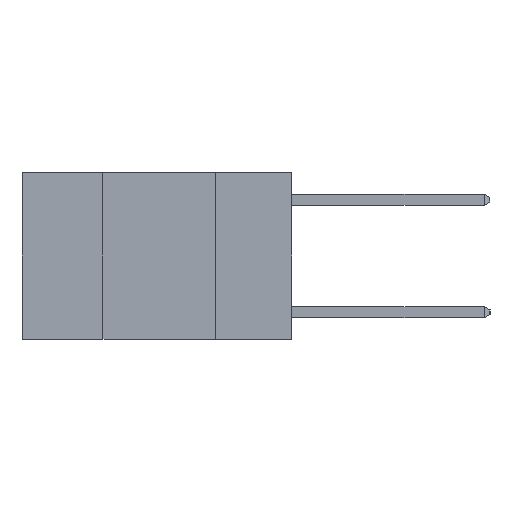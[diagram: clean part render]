
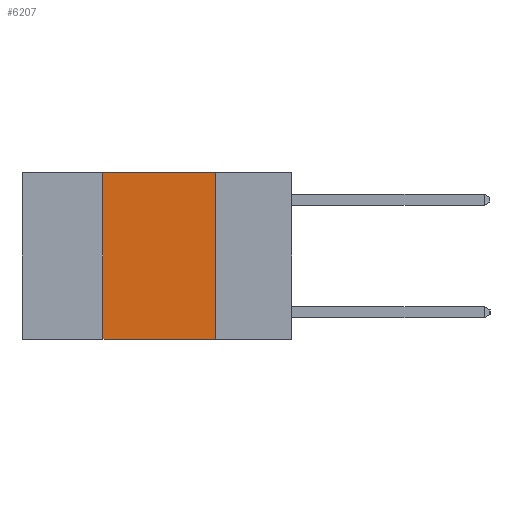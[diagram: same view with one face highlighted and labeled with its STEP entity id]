
A CAD part, left-side view. The second image highlights one B-rep face of the part: STEP entity #6207.
In plain terms, the highlighted planar face has unit normal (-1, 0, 0).
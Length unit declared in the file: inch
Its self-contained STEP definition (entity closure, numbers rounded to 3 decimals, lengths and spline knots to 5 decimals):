
#138 = DIRECTION ( 'NONE',  ( 0., 0., -1. ) ) ;
#323 = EDGE_CURVE ( 'NONE', #2828, #8294, #5029, .T. ) ;
#560 = ORIENTED_EDGE ( 'NONE', *, *, #2396, .F. ) ;
#1161 = LINE ( 'NONE', #9359, #9073 ) ;
#1712 = VERTEX_POINT ( 'NONE', #9080 ) ;
#1921 = VECTOR ( 'NONE', #7247, 39.37008 ) ;
#1958 = DIRECTION ( 'NONE',  ( 0., 0., -1. ) ) ;
#2396 = EDGE_CURVE ( 'NONE', #2738, #1712, #5252, .T. ) ;
#2738 = VERTEX_POINT ( 'NONE', #8018 ) ;
#2828 = VERTEX_POINT ( 'NONE', #9336 ) ;
#2968 = EDGE_CURVE ( 'NONE', #2828, #2738, #4510, .T. ) ;
#3489 = EDGE_CURVE ( 'NONE', #1712, #8294, #1161, .T. ) ;
#3883 = CARTESIAN_POINT ( 'NONE',  ( 0., 0.6, 0. ) ) ;
#4510 = LINE ( 'NONE', #9466, #1921 ) ;
#5029 = LINE ( 'NONE', #9624, #7030 ) ;
#5087 = CARTESIAN_POINT ( 'NONE',  ( 0., 0.6, 0. ) ) ;
#5252 = LINE ( 'NONE', #3883, #8754 ) ;
#6102 = CARTESIAN_POINT ( 'NONE',  ( 0., 0.17, -0.37 ) ) ;
#6207 = ADVANCED_FACE ( 'NONE', ( #9092 ), #8057, .F. ) ;
#6595 = DIRECTION ( 'NONE',  ( 1., 0., 0. ) ) ;
#7030 = VECTOR ( 'NONE', #8127, 39.37008 ) ;
#7241 = AXIS2_PLACEMENT_3D ( 'NONE', #5087, #6595, #1958 ) ;
#7247 = DIRECTION ( 'NONE',  ( 0., 0., 1. ) ) ;
#7663 = DIRECTION ( 'NONE',  ( 0., -1., 0. ) ) ;
#7669 = ORIENTED_EDGE ( 'NONE', *, *, #3489, .F. ) ;
#8018 = CARTESIAN_POINT ( 'NONE',  ( 0., 0.42, 0. ) ) ;
#8057 = PLANE ( 'NONE',  #7241 ) ;
#8127 = DIRECTION ( 'NONE',  ( 0., -1., 0. ) ) ;
#8294 = VERTEX_POINT ( 'NONE', #6102 ) ;
#8510 = ORIENTED_EDGE ( 'NONE', *, *, #323, .T. ) ;
#8754 = VECTOR ( 'NONE', #7663, 39.37008 ) ;
#9073 = VECTOR ( 'NONE', #138, 39.37008 ) ;
#9077 = EDGE_LOOP ( 'NONE', ( #7669, #560, #9791, #8510 ) ) ;
#9080 = CARTESIAN_POINT ( 'NONE',  ( 0., 0.17, 0. ) ) ;
#9092 = FACE_OUTER_BOUND ( 'NONE', #9077, .T. ) ;
#9336 = CARTESIAN_POINT ( 'NONE',  ( 0., 0.42, -0.37 ) ) ;
#9359 = CARTESIAN_POINT ( 'NONE',  ( 0., 0.17, 0. ) ) ;
#9466 = CARTESIAN_POINT ( 'NONE',  ( 0., 0.42, 0. ) ) ;
#9624 = CARTESIAN_POINT ( 'NONE',  ( 0., 0.6, -0.37 ) ) ;
#9791 = ORIENTED_EDGE ( 'NONE', *, *, #2968, .F. ) ;
